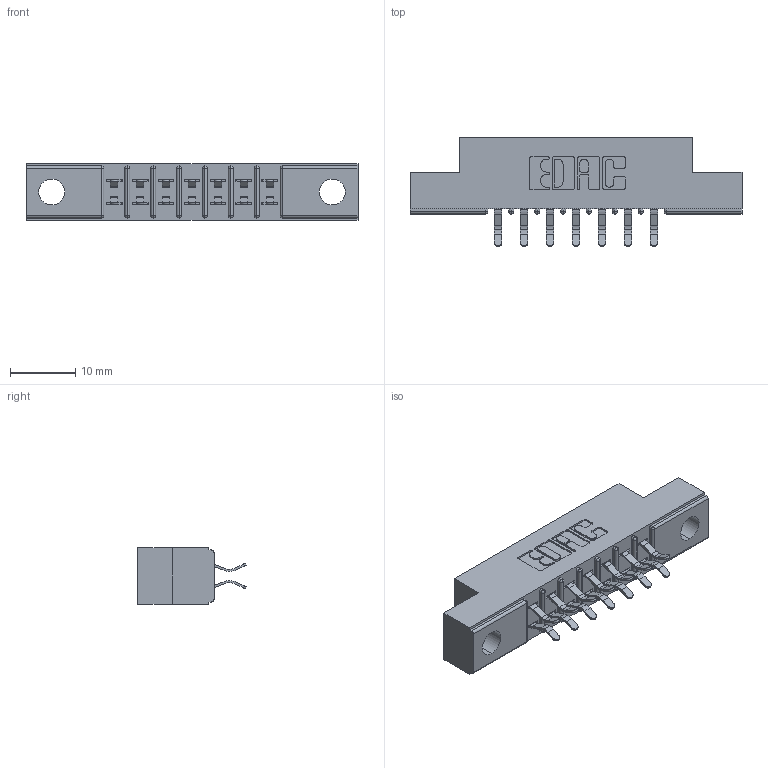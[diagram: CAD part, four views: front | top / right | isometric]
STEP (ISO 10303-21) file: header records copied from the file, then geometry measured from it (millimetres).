
FILE_DESCRIPTION (( 'STEP AP203' ), '1' );
FILE_NAME ('355-014-556-204.STEP', '2019-09-11T01:38:14', ( '' ), ( '' ), 'SwSTEP 2.0', 'SolidWorks 2016', '' );
FILE_SCHEMA (( 'CONFIG_CONTROL_DESIGN' ));
Length unit declared in the file: inch
Products named in the file (3): 305-290-001_556; 305 Part_.156 Dia; 355-014-556-204
Assembly tree (15 placements, depth 2):
  355-014-556-204
    305 Part_.156 Dia
    305-290-001_556  x14
Bounding box: 50.75 x 16.64 x 8.71 mm (x, y, z)
Volume: 3093.6 mm3; surface area: 4877.6 mm2
Topology: 15 solids, 15 shells, 914 faces, 2613 edges, 1702 vertices
Faces by surface type: plane 516, cylinder 370, sphere 28
Entity records: 12480 total; most frequent: CARTESIAN_POINT 2073, ORIENTED_EDGE 2050, DIRECTION 2029, EDGE_CURVE 1025, VECTOR 793, LINE 793, VERTEX_POINT 662, AXIS2_PLACEMENT_3D 618
